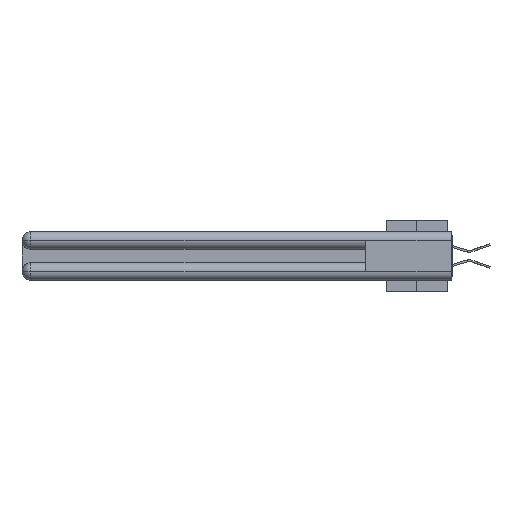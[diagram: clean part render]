
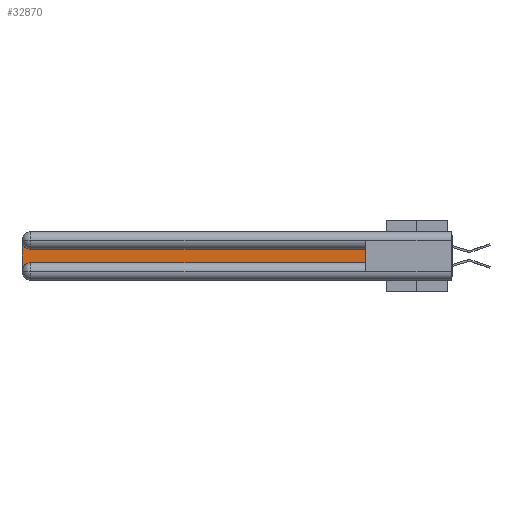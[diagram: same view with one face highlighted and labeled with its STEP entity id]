
A CAD part, left-side view. The second image highlights one B-rep face of the part: STEP entity #32870.
In plain terms, the highlighted planar face has unit normal (-1, 0, 0).
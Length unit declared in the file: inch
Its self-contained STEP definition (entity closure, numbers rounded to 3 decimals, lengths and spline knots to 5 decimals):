
#650 = ORIENTED_EDGE ( 'NONE', *, *, #16273, .T. ) ;
#1578 = EDGE_CURVE ( 'NONE', #28659, #2205, #2338, .T. ) ;
#1735 = VERTEX_POINT ( 'NONE', #3531 ) ;
#2205 = VERTEX_POINT ( 'NONE', #18583 ) ;
#2338 = LINE ( 'NONE', #6690, #10808 ) ;
#2461 = DIRECTION ( 'NONE',  ( 0., 1., 0. ) ) ;
#2540 = VERTEX_POINT ( 'NONE', #26395 ) ;
#2598 = DIRECTION ( 'NONE',  ( 0., 0., -1. ) ) ;
#3531 = CARTESIAN_POINT ( 'NONE',  ( 0.075, 0.6, -0.2175 ) ) ;
#3831 = EDGE_CURVE ( 'NONE', #2205, #31558, #6672, .T. ) ;
#6672 = CIRCLE ( 'NONE', #31233, 0.06 ) ;
#6690 = CARTESIAN_POINT ( 'NONE',  ( 0.075, 3., -0.2175 ) ) ;
#8647 = FACE_OUTER_BOUND ( 'NONE', #34107, .T. ) ;
#9477 = LINE ( 'NONE', #38727, #29226 ) ;
#10808 = VECTOR ( 'NONE', #2598, 39.37008 ) ;
#11264 = DIRECTION ( 'NONE',  ( 0., 0., -1. ) ) ;
#11891 = AXIS2_PLACEMENT_3D ( 'NONE', #40452, #44094, #11264 ) ;
#11923 = DIRECTION ( 'NONE',  ( 0., 0., 1. ) ) ;
#12076 = CARTESIAN_POINT ( 'NONE',  ( 0.075, 0.6, -0.2175 ) ) ;
#13466 = DIRECTION ( 'NONE',  ( 0., 0., -1. ) ) ;
#15426 = VECTOR ( 'NONE', #2461, 39.37008 ) ;
#16068 = CIRCLE ( 'NONE', #11891, 0.06 ) ;
#16273 = EDGE_CURVE ( 'NONE', #1735, #40474, #38137, .T. ) ;
#18583 = CARTESIAN_POINT ( 'NONE',  ( 0.075, 3., -0.2775 ) ) ;
#19548 = EDGE_CURVE ( 'NONE', #40474, #2540, #43631, .T. ) ;
#22438 = AXIS2_PLACEMENT_3D ( 'NONE', #23326, #27069, #23019 ) ;
#23019 = DIRECTION ( 'NONE',  ( 0., 0., -1. ) ) ;
#23326 = CARTESIAN_POINT ( 'NONE',  ( 0.075, 3., -0.1225 ) ) ;
#24692 = EDGE_CURVE ( 'NONE', #2540, #28659, #16068, .T. ) ;
#26377 = CARTESIAN_POINT ( 'NONE',  ( 0.075, 0.6, -0.1225 ) ) ;
#26395 = CARTESIAN_POINT ( 'NONE',  ( 0.075, 2.94, -0.1225 ) ) ;
#26413 = ORIENTED_EDGE ( 'NONE', *, *, #45288, .T. ) ;
#26623 = PLANE ( 'NONE',  #22438 ) ;
#27016 = ORIENTED_EDGE ( 'NONE', *, *, #3831, .T. ) ;
#27069 = DIRECTION ( 'NONE',  ( 1., 0., 0. ) ) ;
#28659 = VERTEX_POINT ( 'NONE', #37302 ) ;
#28872 = ORIENTED_EDGE ( 'NONE', *, *, #1578, .T. ) ;
#29226 = VECTOR ( 'NONE', #39058, 39.37008 ) ;
#30430 = ORIENTED_EDGE ( 'NONE', *, *, #24692, .T. ) ;
#30719 = CARTESIAN_POINT ( 'NONE',  ( 0.075, 0.6, -0.1225 ) ) ;
#31233 = AXIS2_PLACEMENT_3D ( 'NONE', #46159, #39354, #13466 ) ;
#31558 = VERTEX_POINT ( 'NONE', #33075 ) ;
#32821 = ORIENTED_EDGE ( 'NONE', *, *, #19548, .T. ) ;
#32870 = ADVANCED_FACE ( 'NONE', ( #8647 ), #26623, .F. ) ;
#33075 = CARTESIAN_POINT ( 'NONE',  ( 0.075, 2.94, -0.2175 ) ) ;
#34107 = EDGE_LOOP ( 'NONE', ( #32821, #30430, #28872, #27016, #26413, #650 ) ) ;
#37302 = CARTESIAN_POINT ( 'NONE',  ( 0.075, 3., -0.0625 ) ) ;
#38137 = LINE ( 'NONE', #12076, #39289 ) ;
#38727 = CARTESIAN_POINT ( 'NONE',  ( 0.075, 0.6, -0.2175 ) ) ;
#39058 = DIRECTION ( 'NONE',  ( 0., -1., 0. ) ) ;
#39289 = VECTOR ( 'NONE', #11923, 39.37008 ) ;
#39354 = DIRECTION ( 'NONE',  ( 1., 0., 0. ) ) ;
#40452 = CARTESIAN_POINT ( 'NONE',  ( 0.075, 2.94, -0.0625 ) ) ;
#40474 = VERTEX_POINT ( 'NONE', #26377 ) ;
#43631 = LINE ( 'NONE', #30719, #15426 ) ;
#44094 = DIRECTION ( 'NONE',  ( 1., 0., 0. ) ) ;
#45288 = EDGE_CURVE ( 'NONE', #31558, #1735, #9477, .T. ) ;
#46159 = CARTESIAN_POINT ( 'NONE',  ( 0.075, 2.94, -0.2775 ) ) ;
